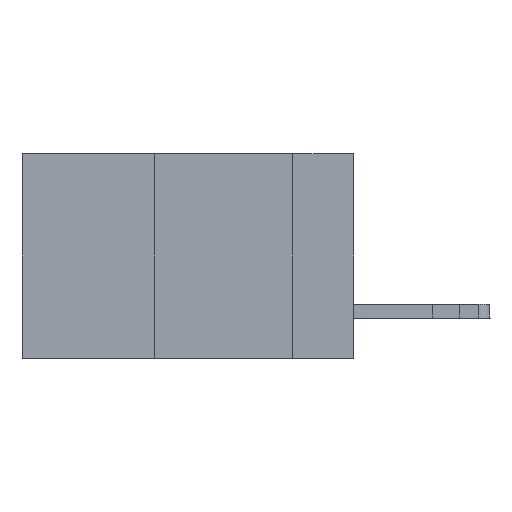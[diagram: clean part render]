
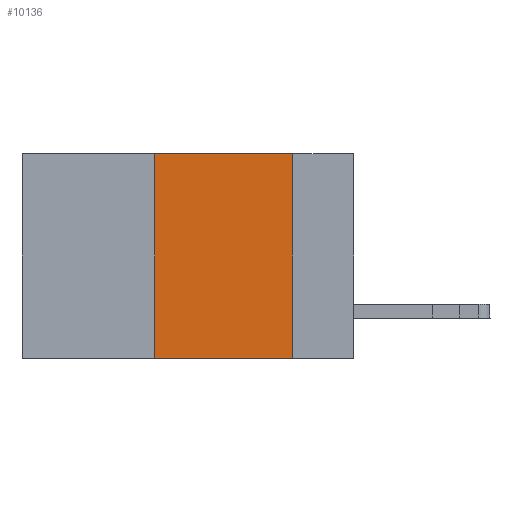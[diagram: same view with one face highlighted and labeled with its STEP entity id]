
A CAD part, left-side view. The second image highlights one B-rep face of the part: STEP entity #10136.
In plain terms, the highlighted planar face has unit normal (-1, 0, 0).
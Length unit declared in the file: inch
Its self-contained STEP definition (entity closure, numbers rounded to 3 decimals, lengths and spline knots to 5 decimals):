
#412 = LINE ( 'NONE', #4854, #1924 ) ;
#820 = DIRECTION ( 'NONE',  ( 0., 0., -1. ) ) ;
#1924 = VECTOR ( 'NONE', #19048, 39.37008 ) ;
#2326 = CARTESIAN_POINT ( 'NONE',  ( 0., 0.11, -0.37 ) ) ;
#2518 = VERTEX_POINT ( 'NONE', #9614 ) ;
#2969 = VECTOR ( 'NONE', #4825, 39.37008 ) ;
#3052 = ORIENTED_EDGE ( 'NONE', *, *, #11116, .F. ) ;
#3498 = VERTEX_POINT ( 'NONE', #2326 ) ;
#4825 = DIRECTION ( 'NONE',  ( 0., -1., 0. ) ) ;
#4854 = CARTESIAN_POINT ( 'NONE',  ( 0., 0.11, 0. ) ) ;
#4962 = CARTESIAN_POINT ( 'NONE',  ( 0., 0.6, -0.37 ) ) ;
#5088 = ORIENTED_EDGE ( 'NONE', *, *, #6127, .T. ) ;
#5155 = EDGE_CURVE ( 'NONE', #2518, #15152, #13570, .T. ) ;
#6127 = EDGE_CURVE ( 'NONE', #2518, #3498, #6827, .T. ) ;
#6280 = DIRECTION ( 'NONE',  ( 0., 0., 1. ) ) ;
#6310 = CARTESIAN_POINT ( 'NONE',  ( 0., 0.36, 0. ) ) ;
#6827 = LINE ( 'NONE', #4962, #2969 ) ;
#7084 = FACE_OUTER_BOUND ( 'NONE', #17345, .T. ) ;
#7106 = DIRECTION ( 'NONE',  ( 0., -1., 0. ) ) ;
#7336 = PLANE ( 'NONE',  #8706 ) ;
#8426 = EDGE_CURVE ( 'NONE', #15152, #16417, #10407, .T. ) ;
#8706 = AXIS2_PLACEMENT_3D ( 'NONE', #19817, #10533, #820 ) ;
#9415 = ORIENTED_EDGE ( 'NONE', *, *, #5155, .F. ) ;
#9614 = CARTESIAN_POINT ( 'NONE',  ( 0., 0.36, -0.37 ) ) ;
#10136 = ADVANCED_FACE ( 'NONE', ( #7084 ), #7336, .F. ) ;
#10407 = LINE ( 'NONE', #16529, #18651 ) ;
#10533 = DIRECTION ( 'NONE',  ( 1., 0., 0. ) ) ;
#11116 = EDGE_CURVE ( 'NONE', #16417, #3498, #412, .T. ) ;
#11885 = ORIENTED_EDGE ( 'NONE', *, *, #8426, .F. ) ;
#12282 = CARTESIAN_POINT ( 'NONE',  ( 0., 0.11, 0. ) ) ;
#13570 = LINE ( 'NONE', #6310, #17200 ) ;
#15152 = VERTEX_POINT ( 'NONE', #19850 ) ;
#16417 = VERTEX_POINT ( 'NONE', #12282 ) ;
#16529 = CARTESIAN_POINT ( 'NONE',  ( 0., 0.6, 0. ) ) ;
#17200 = VECTOR ( 'NONE', #6280, 39.37008 ) ;
#17345 = EDGE_LOOP ( 'NONE', ( #3052, #11885, #9415, #5088 ) ) ;
#18651 = VECTOR ( 'NONE', #7106, 39.37008 ) ;
#19048 = DIRECTION ( 'NONE',  ( 0., 0., -1. ) ) ;
#19817 = CARTESIAN_POINT ( 'NONE',  ( 0., 0.6, 0. ) ) ;
#19850 = CARTESIAN_POINT ( 'NONE',  ( 0., 0.36, 0. ) ) ;
